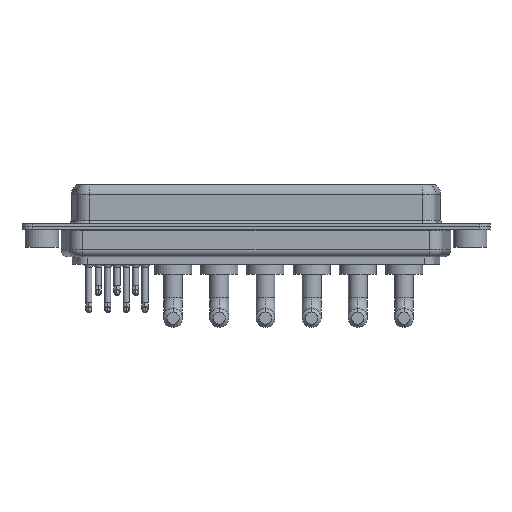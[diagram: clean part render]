
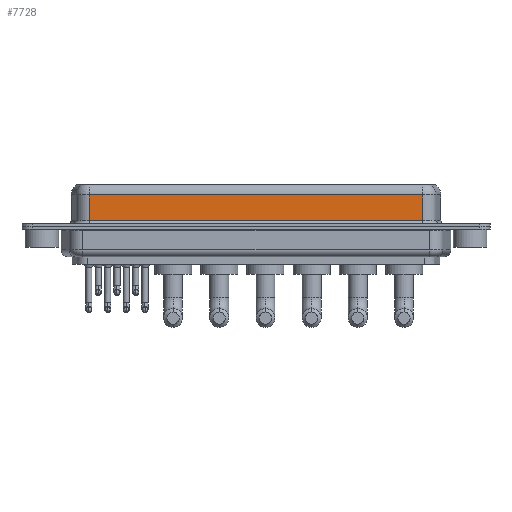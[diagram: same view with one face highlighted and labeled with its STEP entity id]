
A CAD part, front view. The second image highlights one B-rep face of the part: STEP entity #7728.
In plain terms, the highlighted planar face has unit normal (0, -1, 0).
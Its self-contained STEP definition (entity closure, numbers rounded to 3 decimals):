
#468 = CARTESIAN_POINT ( 'NONE',  ( 56.462, -3.95, 6.4 ) ) ;
#519 = VERTEX_POINT ( 'NONE', #5381 ) ;
#582 = CARTESIAN_POINT ( 'NONE',  ( 56.462, -3.95, 4.65 ) ) ;
#909 = VECTOR ( 'NONE', #6876, 1000. ) ;
#1668 = VERTEX_POINT ( 'NONE', #6502 ) ;
#2100 = CARTESIAN_POINT ( 'NONE',  ( 56.462, -3.95, 6.4 ) ) ;
#2132 = EDGE_CURVE ( 'NONE', #1668, #519, #13413, .T. ) ;
#2665 = EDGE_CURVE ( 'NONE', #12090, #1668, #7087, .T. ) ;
#3092 = ORIENTED_EDGE ( 'NONE', *, *, #4540, .T. ) ;
#4050 = ORIENTED_EDGE ( 'NONE', *, *, #2132, .T. ) ;
#4073 = CARTESIAN_POINT ( 'NONE',  ( 56.462, -3.95, 0.9 ) ) ;
#4540 = EDGE_CURVE ( 'NONE', #519, #4650, #18299, .T. ) ;
#4650 = VERTEX_POINT ( 'NONE', #4073 ) ;
#5001 = FACE_OUTER_BOUND ( 'NONE', #16365, .T. ) ;
#5381 = CARTESIAN_POINT ( 'NONE',  ( 7.038, -3.95, 0.9 ) ) ;
#5594 = CARTESIAN_POINT ( 'NONE',  ( 56.462, -3.95, 4.65 ) ) ;
#6184 = DIRECTION ( 'NONE',  ( 0., 0., -1. ) ) ;
#6502 = CARTESIAN_POINT ( 'NONE',  ( 7.038, -3.95, 4.65 ) ) ;
#6876 = DIRECTION ( 'NONE',  ( 1., 0., 0. ) ) ;
#7087 = LINE ( 'NONE', #5594, #14939 ) ;
#7593 = LINE ( 'NONE', #468, #8399 ) ;
#7728 = ADVANCED_FACE ( 'NONE', ( #5001 ), #10936, .F. ) ;
#8069 = DIRECTION ( 'NONE',  ( 0., 0., 1. ) ) ;
#8399 = VECTOR ( 'NONE', #6184, 1000. ) ;
#9861 = DIRECTION ( 'NONE',  ( -1., 0., 0. ) ) ;
#10936 = PLANE ( 'NONE',  #16193 ) ;
#11135 = CARTESIAN_POINT ( 'NONE',  ( 56.462, -3.95, 0.9 ) ) ;
#12090 = VERTEX_POINT ( 'NONE', #582 ) ;
#13295 = ORIENTED_EDGE ( 'NONE', *, *, #16418, .F. ) ;
#13413 = LINE ( 'NONE', #17023, #17587 ) ;
#13425 = DIRECTION ( 'NONE',  ( 0., 1., 0. ) ) ;
#13429 = ORIENTED_EDGE ( 'NONE', *, *, #2665, .T. ) ;
#14939 = VECTOR ( 'NONE', #9861, 1000. ) ;
#16193 = AXIS2_PLACEMENT_3D ( 'NONE', #2100, #13425, #8069 ) ;
#16365 = EDGE_LOOP ( 'NONE', ( #13295, #13429, #4050, #3092 ) ) ;
#16418 = EDGE_CURVE ( 'NONE', #12090, #4650, #7593, .T. ) ;
#17023 = CARTESIAN_POINT ( 'NONE',  ( 7.038, -3.95, 6.4 ) ) ;
#17587 = VECTOR ( 'NONE', #18244, 1000. ) ;
#18244 = DIRECTION ( 'NONE',  ( 0., 0., -1. ) ) ;
#18299 = LINE ( 'NONE', #11135, #909 ) ;
